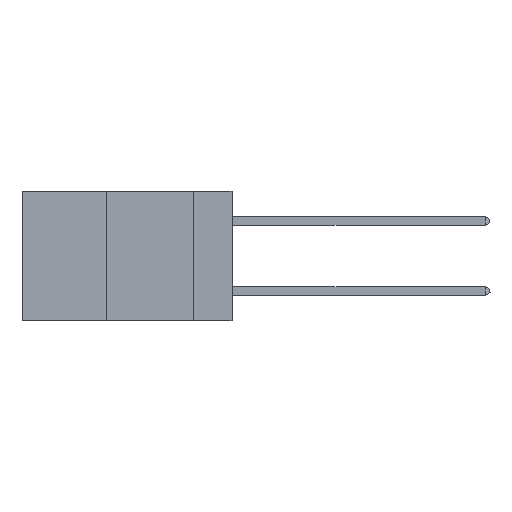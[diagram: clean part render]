
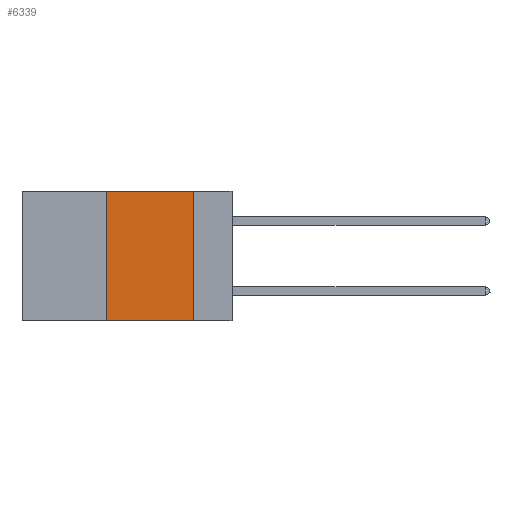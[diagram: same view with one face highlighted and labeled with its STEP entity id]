
A CAD part, left-side view. The second image highlights one B-rep face of the part: STEP entity #6339.
In plain terms, the highlighted planar face has unit normal (-1, 0, 0).
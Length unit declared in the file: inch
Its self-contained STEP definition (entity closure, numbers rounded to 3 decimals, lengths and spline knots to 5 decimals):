
#385 = CARTESIAN_POINT ( 'NONE',  ( 0., 0.36, 0. ) ) ;
#446 = VERTEX_POINT ( 'NONE', #12279 ) ;
#1098 = EDGE_CURVE ( 'NONE', #10953, #2633, #6417, .T. ) ;
#1236 = LINE ( 'NONE', #385, #10127 ) ;
#1253 = DIRECTION ( 'NONE',  ( 0., -1., 0. ) ) ;
#1381 = EDGE_CURVE ( 'NONE', #4772, #446, #1236, .T. ) ;
#1428 = DIRECTION ( 'NONE',  ( 0., 0., 1. ) ) ;
#1463 = ORIENTED_EDGE ( 'NONE', *, *, #10380, .T. ) ;
#2069 = CARTESIAN_POINT ( 'NONE',  ( 0., 0.11, 0. ) ) ;
#2150 = CARTESIAN_POINT ( 'NONE',  ( 0., 0.6, 0. ) ) ;
#2633 = VERTEX_POINT ( 'NONE', #9350 ) ;
#3026 = VECTOR ( 'NONE', #1253, 39.37008 ) ;
#4151 = EDGE_LOOP ( 'NONE', ( #6097, #5485, #7829, #1463 ) ) ;
#4772 = VERTEX_POINT ( 'NONE', #11106 ) ;
#5217 = CARTESIAN_POINT ( 'NONE',  ( 0., 0.11, 0. ) ) ;
#5485 = ORIENTED_EDGE ( 'NONE', *, *, #5684, .F. ) ;
#5684 = EDGE_CURVE ( 'NONE', #446, #10953, #13293, .T. ) ;
#5981 = FACE_OUTER_BOUND ( 'NONE', #4151, .T. ) ;
#6097 = ORIENTED_EDGE ( 'NONE', *, *, #1098, .F. ) ;
#6339 = ADVANCED_FACE ( 'NONE', ( #5981 ), #12185, .F. ) ;
#6417 = LINE ( 'NONE', #2069, #10633 ) ;
#7829 = ORIENTED_EDGE ( 'NONE', *, *, #1381, .F. ) ;
#9350 = CARTESIAN_POINT ( 'NONE',  ( 0., 0.11, -0.37 ) ) ;
#9428 = DIRECTION ( 'NONE',  ( 0., -1., 0. ) ) ;
#9704 = AXIS2_PLACEMENT_3D ( 'NONE', #11194, #12144, #13365 ) ;
#10127 = VECTOR ( 'NONE', #1428, 39.37008 ) ;
#10380 = EDGE_CURVE ( 'NONE', #4772, #2633, #11316, .T. ) ;
#10633 = VECTOR ( 'NONE', #11285, 39.37008 ) ;
#10953 = VERTEX_POINT ( 'NONE', #5217 ) ;
#11106 = CARTESIAN_POINT ( 'NONE',  ( 0., 0.36, -0.37 ) ) ;
#11194 = CARTESIAN_POINT ( 'NONE',  ( 0., 0.6, 0. ) ) ;
#11285 = DIRECTION ( 'NONE',  ( 0., 0., -1. ) ) ;
#11316 = LINE ( 'NONE', #12817, #3026 ) ;
#11345 = VECTOR ( 'NONE', #9428, 39.37008 ) ;
#12144 = DIRECTION ( 'NONE',  ( 1., 0., 0. ) ) ;
#12185 = PLANE ( 'NONE',  #9704 ) ;
#12279 = CARTESIAN_POINT ( 'NONE',  ( 0., 0.36, 0. ) ) ;
#12817 = CARTESIAN_POINT ( 'NONE',  ( 0., 0.6, -0.37 ) ) ;
#13293 = LINE ( 'NONE', #2150, #11345 ) ;
#13365 = DIRECTION ( 'NONE',  ( 0., 0., -1. ) ) ;
